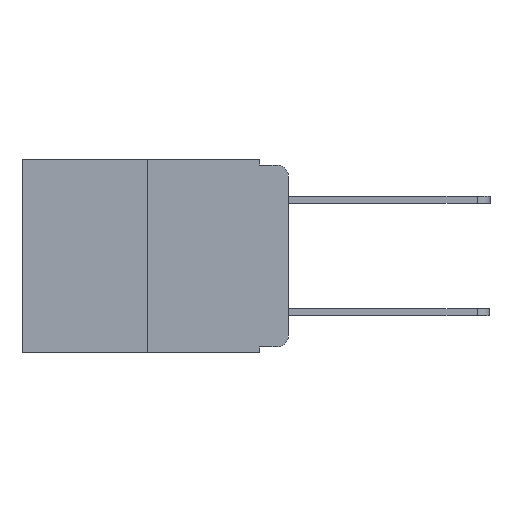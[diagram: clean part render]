
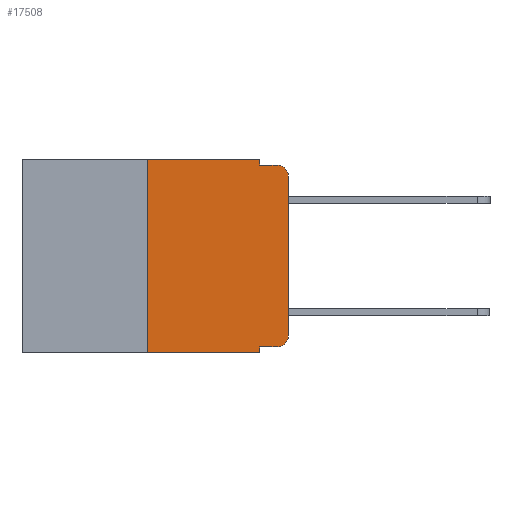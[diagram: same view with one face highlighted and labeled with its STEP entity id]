
A CAD part, left-side view. The second image highlights one B-rep face of the part: STEP entity #17508.
In plain terms, the highlighted planar face has unit normal (-1, 0, 0).
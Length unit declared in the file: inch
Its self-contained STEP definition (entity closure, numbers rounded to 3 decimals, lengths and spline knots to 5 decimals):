
#182 = CARTESIAN_POINT ( 'NONE',  ( 0., 0.051, -0.01 ) ) ;
#994 = VECTOR ( 'NONE', #22591, 39.37008 ) ;
#1707 = EDGE_CURVE ( 'NONE', #3565, #2628, #19632, .T. ) ;
#1923 = VECTOR ( 'NONE', #14494, 39.37008 ) ;
#1931 = EDGE_CURVE ( 'NONE', #14444, #4185, #15669, .T. ) ;
#2089 = CARTESIAN_POINT ( 'NONE',  ( 0., 0.051, 0. ) ) ;
#2555 = CARTESIAN_POINT ( 'NONE',  ( 0., 0.02, -0.03 ) ) ;
#2628 = VERTEX_POINT ( 'NONE', #9939 ) ;
#3336 = CARTESIAN_POINT ( 'NONE',  ( 0., 0.02, -0.01 ) ) ;
#3565 = VERTEX_POINT ( 'NONE', #6682 ) ;
#4145 = DIRECTION ( 'NONE',  ( 0., -1., 0. ) ) ;
#4149 = DIRECTION ( 'NONE',  ( 0., 0., 1. ) ) ;
#4150 = ORIENTED_EDGE ( 'NONE', *, *, #20147, .F. ) ;
#4185 = VERTEX_POINT ( 'NONE', #6285 ) ;
#4230 = CARTESIAN_POINT ( 'NONE',  ( 0., 0., 0. ) ) ;
#4521 = DIRECTION ( 'NONE',  ( 0., 0., -1. ) ) ;
#4523 = EDGE_CURVE ( 'NONE', #21485, #22774, #20914, .T. ) ;
#4888 = VECTOR ( 'NONE', #19866, 39.37008 ) ;
#5824 = CIRCLE ( 'NONE', #15440, 0.02 ) ;
#5964 = CARTESIAN_POINT ( 'NONE',  ( 0., 0.051, -0.333 ) ) ;
#6285 = CARTESIAN_POINT ( 'NONE',  ( 0., 0.051, -0.343 ) ) ;
#6322 = VERTEX_POINT ( 'NONE', #18787 ) ;
#6408 = FACE_OUTER_BOUND ( 'NONE', #11002, .T. ) ;
#6572 = DIRECTION ( 'NONE',  ( -1., 0., 0. ) ) ;
#6682 = CARTESIAN_POINT ( 'NONE',  ( 0., 0.25, -0.343 ) ) ;
#6742 = CARTESIAN_POINT ( 'NONE',  ( 0., 0.051, -0.01 ) ) ;
#7329 = AXIS2_PLACEMENT_3D ( 'NONE', #2555, #15544, #4521 ) ;
#7379 = LINE ( 'NONE', #13653, #994 ) ;
#7727 = CIRCLE ( 'NONE', #7329, 0.02 ) ;
#8398 = VERTEX_POINT ( 'NONE', #16141 ) ;
#8772 = EDGE_CURVE ( 'NONE', #22774, #21196, #7727, .T. ) ;
#9446 = ORIENTED_EDGE ( 'NONE', *, *, #11691, .T. ) ;
#9751 = ORIENTED_EDGE ( 'NONE', *, *, #8772, .T. ) ;
#9939 = CARTESIAN_POINT ( 'NONE',  ( 0., 0.25, 0. ) ) ;
#11002 = EDGE_LOOP ( 'NONE', ( #18263, #9751, #4150, #15145, #16844, #20487, #21593, #22701, #12017, #9446 ) ) ;
#11110 = PLANE ( 'NONE',  #22448 ) ;
#11429 = DIRECTION ( 'NONE',  ( 0., 0., -1. ) ) ;
#11691 = EDGE_CURVE ( 'NONE', #6322, #21485, #5824, .T. ) ;
#11965 = DIRECTION ( 'NONE',  ( 0., -1., 0. ) ) ;
#12017 = ORIENTED_EDGE ( 'NONE', *, *, #23752, .T. ) ;
#12510 = LINE ( 'NONE', #19932, #1923 ) ;
#12926 = DIRECTION ( 'NONE',  ( 0., 0., -1. ) ) ;
#13102 = CARTESIAN_POINT ( 'NONE',  ( 0., 0., -0.03 ) ) ;
#13317 = CARTESIAN_POINT ( 'NONE',  ( 0., 0.25, 0. ) ) ;
#13352 = EDGE_CURVE ( 'NONE', #8398, #15929, #7379, .T. ) ;
#13653 = CARTESIAN_POINT ( 'NONE',  ( 0., 0.051, 0. ) ) ;
#13809 = VECTOR ( 'NONE', #4145, 39.37008 ) ;
#14376 = LINE ( 'NONE', #182, #13809 ) ;
#14444 = VERTEX_POINT ( 'NONE', #5964 ) ;
#14494 = DIRECTION ( 'NONE',  ( 0., -1., 0. ) ) ;
#14497 = CARTESIAN_POINT ( 'NONE',  ( 0., 0.473, -0.343 ) ) ;
#14831 = VECTOR ( 'NONE', #4149, 39.37008 ) ;
#15145 = ORIENTED_EDGE ( 'NONE', *, *, #13352, .F. ) ;
#15188 = EDGE_CURVE ( 'NONE', #2628, #8398, #19246, .T. ) ;
#15240 = LINE ( 'NONE', #14497, #4888 ) ;
#15286 = DIRECTION ( 'NONE',  ( 0., 0., 1. ) ) ;
#15440 = AXIS2_PLACEMENT_3D ( 'NONE', #17517, #6572, #19325 ) ;
#15544 = DIRECTION ( 'NONE',  ( -1., 0., 0. ) ) ;
#15669 = LINE ( 'NONE', #2089, #17956 ) ;
#15929 = VERTEX_POINT ( 'NONE', #6742 ) ;
#16141 = CARTESIAN_POINT ( 'NONE',  ( 0., 0.051, 0. ) ) ;
#16171 = VECTOR ( 'NONE', #15286, 39.37008 ) ;
#16844 = ORIENTED_EDGE ( 'NONE', *, *, #15188, .F. ) ;
#17508 = ADVANCED_FACE ( 'NONE', ( #6408 ), #11110, .F. ) ;
#17517 = CARTESIAN_POINT ( 'NONE',  ( 0., 0.02, -0.313 ) ) ;
#17956 = VECTOR ( 'NONE', #11429, 39.37008 ) ;
#18263 = ORIENTED_EDGE ( 'NONE', *, *, #4523, .T. ) ;
#18787 = CARTESIAN_POINT ( 'NONE',  ( 0., 0.02, -0.333 ) ) ;
#19246 = LINE ( 'NONE', #22760, #23421 ) ;
#19325 = DIRECTION ( 'NONE',  ( 0., 0., -1. ) ) ;
#19632 = LINE ( 'NONE', #13317, #14831 ) ;
#19866 = DIRECTION ( 'NONE',  ( 0., -1., 0. ) ) ;
#19896 = EDGE_CURVE ( 'NONE', #3565, #4185, #15240, .T. ) ;
#19932 = CARTESIAN_POINT ( 'NONE',  ( 0., 0.051, -0.333 ) ) ;
#20147 = EDGE_CURVE ( 'NONE', #15929, #21196, #14376, .T. ) ;
#20487 = ORIENTED_EDGE ( 'NONE', *, *, #1707, .F. ) ;
#20704 = CARTESIAN_POINT ( 'NONE',  ( 0., 0., -0.313 ) ) ;
#20914 = LINE ( 'NONE', #4230, #16171 ) ;
#21196 = VERTEX_POINT ( 'NONE', #3336 ) ;
#21485 = VERTEX_POINT ( 'NONE', #20704 ) ;
#21593 = ORIENTED_EDGE ( 'NONE', *, *, #19896, .T. ) ;
#21897 = CARTESIAN_POINT ( 'NONE',  ( 0., 0.473, 0. ) ) ;
#22448 = AXIS2_PLACEMENT_3D ( 'NONE', #21897, #23694, #12926 ) ;
#22591 = DIRECTION ( 'NONE',  ( 0., 0., -1. ) ) ;
#22701 = ORIENTED_EDGE ( 'NONE', *, *, #1931, .F. ) ;
#22760 = CARTESIAN_POINT ( 'NONE',  ( 0., 0.473, 0. ) ) ;
#22774 = VERTEX_POINT ( 'NONE', #13102 ) ;
#23421 = VECTOR ( 'NONE', #11965, 39.37008 ) ;
#23694 = DIRECTION ( 'NONE',  ( 1., 0., 0. ) ) ;
#23752 = EDGE_CURVE ( 'NONE', #14444, #6322, #12510, .T. ) ;
